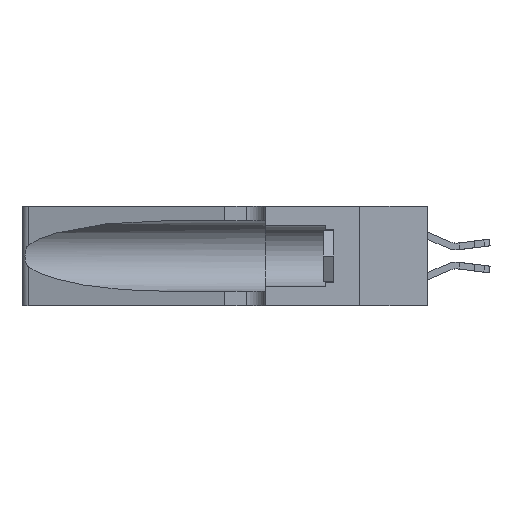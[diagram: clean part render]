
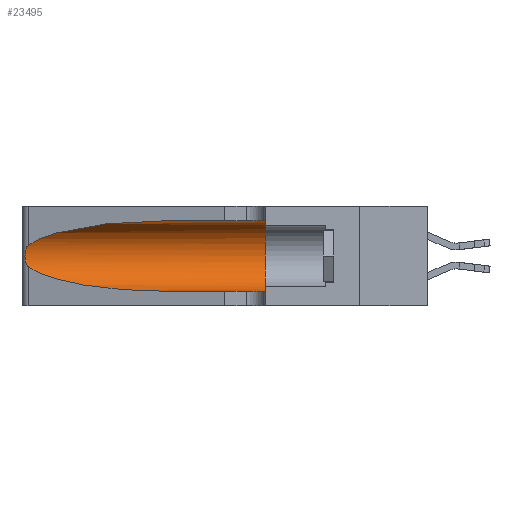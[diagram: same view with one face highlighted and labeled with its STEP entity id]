
A CAD part, left-side view. The second image highlights one B-rep face of the part: STEP entity #23495.
In plain terms, the highlighted cylindrical face has radius 3.308 mm (diameter 6.617 mm), a partial arc.
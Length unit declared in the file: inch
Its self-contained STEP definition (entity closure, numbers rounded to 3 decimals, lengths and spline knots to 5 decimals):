
#151 = CARTESIAN_POINT ( 'NONE',  ( 0.26075, 1.23896, 0.19203 ) ) ;
#540 = ORIENTED_EDGE ( 'NONE', *, *, #12587, .T. ) ;
#903 = VERTEX_POINT ( 'NONE', #9862 ) ;
#974 = DIRECTION ( 'NONE',  ( 0., -1., 0. ) ) ;
#1226 = CARTESIAN_POINT ( 'NONE',  ( 0.1305, 0.35, 0.31525 ) ) ;
#1868 = DIRECTION ( 'NONE',  ( 0., 0., -1. ) ) ;
#2607 = CYLINDRICAL_SURFACE ( 'NONE', #24550, 0.13025 ) ;
#2765 = EDGE_CURVE ( 'NONE', #8731, #16272, #6317, .T. ) ;
#3062 = LINE ( 'NONE', #3874, #11675 ) ;
#3330 = FACE_OUTER_BOUND ( 'NONE', #15061, .T. ) ;
#3874 = CARTESIAN_POINT ( 'NONE',  ( 0.1305, 1.61858, 0.31525 ) ) ;
#4085 = CARTESIAN_POINT ( 'NONE',  ( 0.26018, 1.23835, 0.19895 ) ) ;
#4132 = CARTESIAN_POINT ( 'NONE',  ( 0.1305, 0.72297, 0.05475 ) ) ;
#4366 =( BOUNDED_CURVE ( )  B_SPLINE_CURVE ( 3, ( #6160, #24287, #6071, #16205 ),
 .UNSPECIFIED., .F., .F. ) 
 B_SPLINE_CURVE_WITH_KNOTS ( ( 4, 4 ),
 ( 1.5708, 2.84003 ),
 .UNSPECIFIED. ) 
 CURVE ( )  GEOMETRIC_REPRESENTATION_ITEM ( )  RATIONAL_B_SPLINE_CURVE ( ( 1., 0.87, 0.87, 1. ) ) 
 REPRESENTATION_ITEM ( '' )  );
#4600 = EDGE_CURVE ( 'NONE', #21936, #16272, #19038, .T. ) ;
#4922 = EDGE_CURVE ( 'NONE', #11348, #24348, #19669, .T. ) ;
#6071 = CARTESIAN_POINT ( 'NONE',  ( 0.2373, 1.15595, 0.28018 ) ) ;
#6118 = CARTESIAN_POINT ( 'NONE',  ( 0.26017, 1.23833, 0.17102 ) ) ;
#6160 = CARTESIAN_POINT ( 'NONE',  ( 0.1305, 0.72297, 0.31525 ) ) ;
#6317 = LINE ( 'NONE', #19307, #17446 ) ;
#8247 = CARTESIAN_POINT ( 'NONE',  ( 0.25789, 1.23486, 0.15765 ) ) ;
#8731 = VERTEX_POINT ( 'NONE', #4132 ) ;
#9130 = CARTESIAN_POINT ( 'NONE',  ( 0.25487, 1.22718, 0.14631 ) ) ;
#9299 = EDGE_CURVE ( 'NONE', #24348, #8731, #12182, .T. ) ;
#9302 = AXIS2_PLACEMENT_3D ( 'NONE', #15071, #17150, #11205 ) ;
#9484 = CARTESIAN_POINT ( 'NONE',  ( 0.18966, 0.96281, 0.05475 ) ) ;
#9862 = CARTESIAN_POINT ( 'NONE',  ( 0.1305, 0.72297, 0.31525 ) ) ;
#10298 = CARTESIAN_POINT ( 'NONE',  ( 0.25639, 1.23186, 0.15144 ) ) ;
#11102 = CARTESIAN_POINT ( 'NONE',  ( 0.25487, 1.22718, 0.22369 ) ) ;
#11205 = DIRECTION ( 'NONE',  ( 0., 0., 1. ) ) ;
#11348 = VERTEX_POINT ( 'NONE', #18293 ) ;
#11675 = VECTOR ( 'NONE', #18106, 39.37008 ) ;
#12182 =( BOUNDED_CURVE ( )  B_SPLINE_CURVE ( 3, ( #15861, #25760, #9484, #17860 ),
 .UNSPECIFIED., .F., .F. ) 
 B_SPLINE_CURVE_WITH_KNOTS ( ( 4, 4 ),
 ( 3.44316, 4.71239 ),
 .UNSPECIFIED. ) 
 CURVE ( )  GEOMETRIC_REPRESENTATION_ITEM ( )  RATIONAL_B_SPLINE_CURVE ( ( 1., 0.87, 0.87, 1. ) ) 
 REPRESENTATION_ITEM ( '' )  );
#12587 = EDGE_CURVE ( 'NONE', #903, #11348, #4366, .T. ) ;
#13578 = ORIENTED_EDGE ( 'NONE', *, *, #9299, .T. ) ;
#15044 = CARTESIAN_POINT ( 'NONE',  ( 0.25787, 1.23484, 0.2124 ) ) ;
#15061 = EDGE_LOOP ( 'NONE', ( #540, #15492, #13578, #15283, #17658, #24218 ) ) ;
#15071 = CARTESIAN_POINT ( 'NONE',  ( 0.1305, 0.35, 0.185 ) ) ;
#15218 = CARTESIAN_POINT ( 'NONE',  ( 0.25639, 1.23184, 0.21858 ) ) ;
#15283 = ORIENTED_EDGE ( 'NONE', *, *, #2765, .T. ) ;
#15492 = ORIENTED_EDGE ( 'NONE', *, *, #4922, .T. ) ;
#15861 = CARTESIAN_POINT ( 'NONE',  ( 0.25487, 1.22718, 0.14631 ) ) ;
#16205 = CARTESIAN_POINT ( 'NONE',  ( 0.25487, 1.22718, 0.22369 ) ) ;
#16272 = VERTEX_POINT ( 'NONE', #21821 ) ;
#17150 = DIRECTION ( 'NONE',  ( 0., 1., 0. ) ) ;
#17446 = VECTOR ( 'NONE', #974, 39.37008 ) ;
#17658 = ORIENTED_EDGE ( 'NONE', *, *, #4600, .F. ) ;
#17860 = CARTESIAN_POINT ( 'NONE',  ( 0.1305, 0.72297, 0.05475 ) ) ;
#18106 = DIRECTION ( 'NONE',  ( 0., -1., 0. ) ) ;
#18268 = EDGE_CURVE ( 'NONE', #903, #21936, #3062, .T. ) ;
#18293 = CARTESIAN_POINT ( 'NONE',  ( 0.25487, 1.22718, 0.22369 ) ) ;
#18307 = CARTESIAN_POINT ( 'NONE',  ( 0.26075, 1.23896, 0.178 ) ) ;
#18570 = CARTESIAN_POINT ( 'NONE',  ( 0.25487, 1.22718, 0.14631 ) ) ;
#19038 = CIRCLE ( 'NONE', #9302, 0.13025 ) ;
#19307 = CARTESIAN_POINT ( 'NONE',  ( 0.1305, 1.61858, 0.05475 ) ) ;
#19669 = B_SPLINE_CURVE_WITH_KNOTS ( 'NONE', 3,
 ( #11102, #25224, #15218, #15044, #22486, #4085, #151, #18307, #6118, #20334, #8247, #10298, #24603, #18570 ),
 .UNSPECIFIED., .F., .F.,
 ( 4, 2, 2, 2, 2, 2, 4 ),
 ( 0., 0.00027, 0.00053, 0.00107, 0.0016, 0.00187, 0.00214 ),
 .UNSPECIFIED. ) ;
#20097 = CARTESIAN_POINT ( 'NONE',  ( 0.1305, 1.61858, 0.185 ) ) ;
#20334 = CARTESIAN_POINT ( 'NONE',  ( 0.25856, 1.23593, 0.16098 ) ) ;
#21821 = CARTESIAN_POINT ( 'NONE',  ( 0.1305, 0.35, 0.05475 ) ) ;
#21936 = VERTEX_POINT ( 'NONE', #1226 ) ;
#22156 = DIRECTION ( 'NONE',  ( 0., -1., 0. ) ) ;
#22486 = CARTESIAN_POINT ( 'NONE',  ( 0.25854, 1.2359, 0.20912 ) ) ;
#23495 = ADVANCED_FACE ( 'NONE', ( #3330 ), #2607, .F. ) ;
#24218 = ORIENTED_EDGE ( 'NONE', *, *, #18268, .F. ) ;
#24287 = CARTESIAN_POINT ( 'NONE',  ( 0.18966, 0.96281, 0.31525 ) ) ;
#24348 = VERTEX_POINT ( 'NONE', #9130 ) ;
#24550 = AXIS2_PLACEMENT_3D ( 'NONE', #20097, #22156, #1868 ) ;
#24603 = CARTESIAN_POINT ( 'NONE',  ( 0.25555, 1.22993, 0.14849 ) ) ;
#25224 = CARTESIAN_POINT ( 'NONE',  ( 0.25555, 1.22994, 0.2215 ) ) ;
#25760 = CARTESIAN_POINT ( 'NONE',  ( 0.2373, 1.15595, 0.08982 ) ) ;
